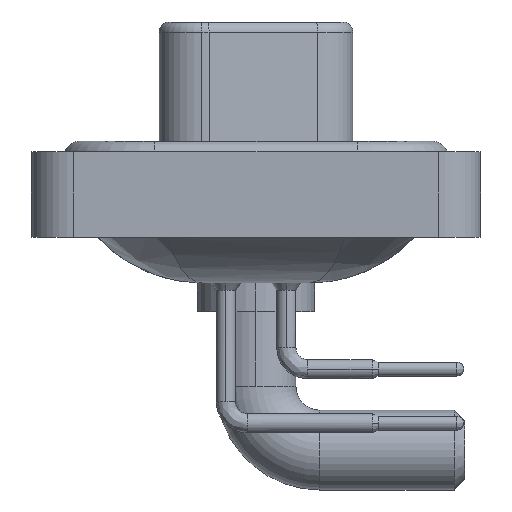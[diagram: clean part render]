
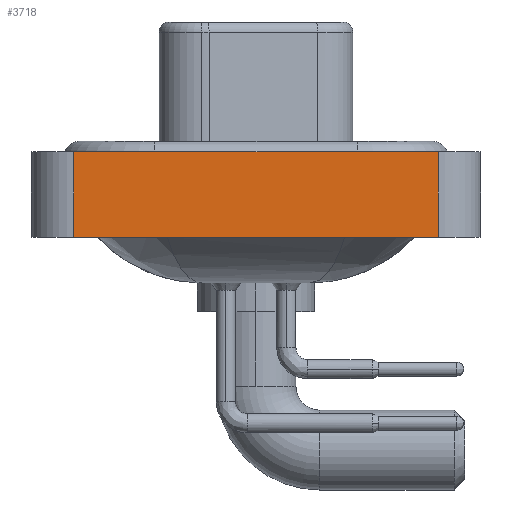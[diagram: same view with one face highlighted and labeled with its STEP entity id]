
A CAD part, left-side view. The second image highlights one B-rep face of the part: STEP entity #3718.
In plain terms, the highlighted planar face has unit normal (-1, 0, 0).
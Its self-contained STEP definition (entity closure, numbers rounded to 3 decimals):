
#587 = VECTOR ( 'NONE', #7059, 1000. ) ;
#1607 = CARTESIAN_POINT ( 'NONE',  ( -7.25, 8.55, -3.6 ) ) ;
#2616 = ORIENTED_EDGE ( 'NONE', *, *, #4409, .T. ) ;
#3718 = ADVANCED_FACE ( 'NONE', ( #11480 ), #7375, .T. ) ;
#4409 = EDGE_CURVE ( 'NONE', #7560, #22073, #15501, .T. ) ;
#4488 = CARTESIAN_POINT ( 'NONE',  ( -7.25, -8.55, 0.4 ) ) ;
#4888 = DIRECTION ( 'NONE',  ( 0., 0., 1. ) ) ;
#5370 = CARTESIAN_POINT ( 'NONE',  ( -7.25, -8.55, -3.6 ) ) ;
#6951 = CARTESIAN_POINT ( 'NONE',  ( -7.25, -8.55, -3.6 ) ) ;
#7059 = DIRECTION ( 'NONE',  ( 0., -1., 0. ) ) ;
#7375 = PLANE ( 'NONE',  #9464 ) ;
#7560 = VERTEX_POINT ( 'NONE', #9696 ) ;
#8707 = DIRECTION ( 'NONE',  ( 0., 0., 1. ) ) ;
#8715 = ORIENTED_EDGE ( 'NONE', *, *, #11439, .T. ) ;
#9464 = AXIS2_PLACEMENT_3D ( 'NONE', #19636, #9537, #9760 ) ;
#9537 = DIRECTION ( 'NONE',  ( -1., 0., 0. ) ) ;
#9696 = CARTESIAN_POINT ( 'NONE',  ( -7.25, 8.55, -3.6 ) ) ;
#9758 = ORIENTED_EDGE ( 'NONE', *, *, #13330, .F. ) ;
#9760 = DIRECTION ( 'NONE',  ( 0., 0., 1. ) ) ;
#10435 = LINE ( 'NONE', #1607, #21783 ) ;
#11038 = ORIENTED_EDGE ( 'NONE', *, *, #12309, .F. ) ;
#11439 = EDGE_CURVE ( 'NONE', #22073, #14985, #14034, .T. ) ;
#11480 = FACE_OUTER_BOUND ( 'NONE', #15577, .T. ) ;
#11556 = DIRECTION ( 'NONE',  ( 0., -1., 0. ) ) ;
#12309 = EDGE_CURVE ( 'NONE', #17155, #14985, #20364, .T. ) ;
#13330 = EDGE_CURVE ( 'NONE', #7560, #17155, #10435, .T. ) ;
#14034 = LINE ( 'NONE', #20883, #19070 ) ;
#14985 = VERTEX_POINT ( 'NONE', #20952 ) ;
#15501 = LINE ( 'NONE', #6951, #587 ) ;
#15577 = EDGE_LOOP ( 'NONE', ( #8715, #11038, #9758, #2616 ) ) ;
#15868 = CARTESIAN_POINT ( 'NONE',  ( -7.25, 8.55, 0.4 ) ) ;
#17155 = VERTEX_POINT ( 'NONE', #15868 ) ;
#17605 = VECTOR ( 'NONE', #11556, 1000. ) ;
#19070 = VECTOR ( 'NONE', #4888, 1000. ) ;
#19636 = CARTESIAN_POINT ( 'NONE',  ( -7.25, -8.55, -3.6 ) ) ;
#20364 = LINE ( 'NONE', #4488, #17605 ) ;
#20883 = CARTESIAN_POINT ( 'NONE',  ( -7.25, -8.55, -3.6 ) ) ;
#20952 = CARTESIAN_POINT ( 'NONE',  ( -7.25, -8.55, 0.4 ) ) ;
#21783 = VECTOR ( 'NONE', #8707, 1000. ) ;
#22073 = VERTEX_POINT ( 'NONE', #5370 ) ;
